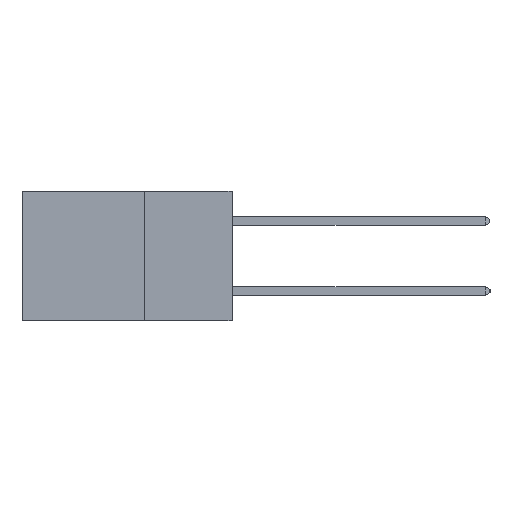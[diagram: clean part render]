
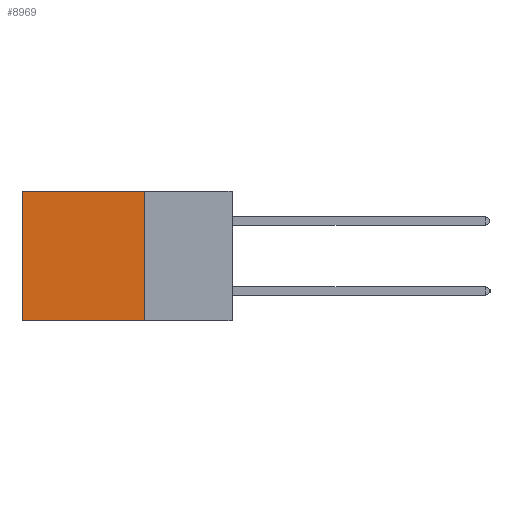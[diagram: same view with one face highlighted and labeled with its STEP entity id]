
A CAD part, left-side view. The second image highlights one B-rep face of the part: STEP entity #8969.
In plain terms, the highlighted planar face has unit normal (-1, 0, 0).
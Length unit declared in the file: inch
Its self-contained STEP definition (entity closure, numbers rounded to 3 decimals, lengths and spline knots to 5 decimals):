
#1540 = LINE ( 'NONE', #18036, #18415 ) ;
#1975 = VERTEX_POINT ( 'NONE', #9725 ) ;
#3088 = LINE ( 'NONE', #10341, #19868 ) ;
#3983 = CARTESIAN_POINT ( 'NONE',  ( 0.2875, 0.25, 0. ) ) ;
#4238 = VERTEX_POINT ( 'NONE', #13457 ) ;
#5259 = ORIENTED_EDGE ( 'NONE', *, *, #18811, .T. ) ;
#6295 = FACE_OUTER_BOUND ( 'NONE', #10227, .T. ) ;
#6991 = AXIS2_PLACEMENT_3D ( 'NONE', #3983, #17498, #7407 ) ;
#7407 = DIRECTION ( 'NONE',  ( 0., 0., -1. ) ) ;
#8265 = LINE ( 'NONE', #15749, #12295 ) ;
#8724 = CARTESIAN_POINT ( 'NONE',  ( 0.2875, 0.25, -0.37 ) ) ;
#8814 = VERTEX_POINT ( 'NONE', #10337 ) ;
#8969 = ADVANCED_FACE ( 'NONE', ( #6295 ), #15904, .F. ) ;
#9436 = CARTESIAN_POINT ( 'NONE',  ( 0.2875, 0.25, 0. ) ) ;
#9712 = DIRECTION ( 'NONE',  ( 0., 0., -1. ) ) ;
#9725 = CARTESIAN_POINT ( 'NONE',  ( 0.2875, 0.25, 0. ) ) ;
#9743 = EDGE_CURVE ( 'NONE', #1975, #15091, #1540, .T. ) ;
#10227 = EDGE_LOOP ( 'NONE', ( #20644, #20894, #17531, #5259 ) ) ;
#10337 = CARTESIAN_POINT ( 'NONE',  ( 0.2875, 0.6, -0.37 ) ) ;
#10341 = CARTESIAN_POINT ( 'NONE',  ( 0.2875, 0.6, 0. ) ) ;
#10475 = EDGE_CURVE ( 'NONE', #4238, #8814, #3088, .T. ) ;
#12106 = DIRECTION ( 'NONE',  ( 0., 0., -1. ) ) ;
#12295 = VECTOR ( 'NONE', #17344, 39.37008 ) ;
#13457 = CARTESIAN_POINT ( 'NONE',  ( 0.2875, 0.6, 0. ) ) ;
#14541 = EDGE_CURVE ( 'NONE', #15091, #8814, #8265, .T. ) ;
#15091 = VERTEX_POINT ( 'NONE', #8724 ) ;
#15749 = CARTESIAN_POINT ( 'NONE',  ( 0.2875, 0.25, -0.37 ) ) ;
#15904 = PLANE ( 'NONE',  #6991 ) ;
#15978 = LINE ( 'NONE', #9436, #19703 ) ;
#17344 = DIRECTION ( 'NONE',  ( 0., 1., 0. ) ) ;
#17498 = DIRECTION ( 'NONE',  ( 1., 0., 0. ) ) ;
#17531 = ORIENTED_EDGE ( 'NONE', *, *, #9743, .F. ) ;
#18036 = CARTESIAN_POINT ( 'NONE',  ( 0.2875, 0.25, 0. ) ) ;
#18415 = VECTOR ( 'NONE', #9712, 39.37008 ) ;
#18811 = EDGE_CURVE ( 'NONE', #1975, #4238, #15978, .T. ) ;
#19358 = DIRECTION ( 'NONE',  ( 0., 1., 0. ) ) ;
#19703 = VECTOR ( 'NONE', #19358, 39.37008 ) ;
#19868 = VECTOR ( 'NONE', #12106, 39.37008 ) ;
#20644 = ORIENTED_EDGE ( 'NONE', *, *, #10475, .T. ) ;
#20894 = ORIENTED_EDGE ( 'NONE', *, *, #14541, .F. ) ;
